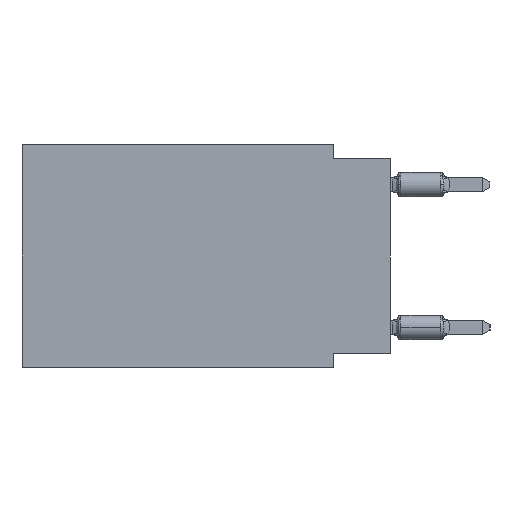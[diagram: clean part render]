
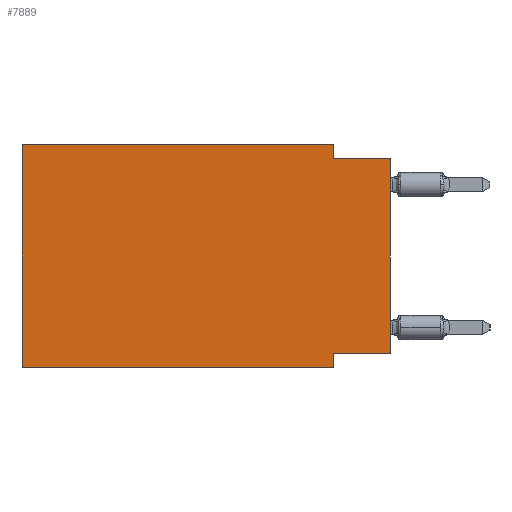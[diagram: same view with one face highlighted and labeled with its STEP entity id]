
A CAD part, left-side view. The second image highlights one B-rep face of the part: STEP entity #7889.
In plain terms, the highlighted planar face has unit normal (-1, 0, 0).
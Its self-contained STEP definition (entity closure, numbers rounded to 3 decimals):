
#257 = LINE ( 'NONE', #14375, #17626 ) ;
#708 = ORIENTED_EDGE ( 'NONE', *, *, #10401, .F. ) ;
#762 = CARTESIAN_POINT ( 'NONE',  ( 0., 16.383, 0. ) ) ;
#1144 = CARTESIAN_POINT ( 'NONE',  ( 0., 0., -9.271 ) ) ;
#1500 = LINE ( 'NONE', #25648, #29223 ) ;
#1559 = DIRECTION ( 'NONE',  ( 0., 0., -1. ) ) ;
#2504 = VERTEX_POINT ( 'NONE', #33860 ) ;
#2645 = VERTEX_POINT ( 'NONE', #31160 ) ;
#3160 = ORIENTED_EDGE ( 'NONE', *, *, #23300, .T. ) ;
#3609 = EDGE_CURVE ( 'NONE', #29315, #2645, #22006, .T. ) ;
#3831 = CARTESIAN_POINT ( 'NONE',  ( 0., 2.54, -9.906 ) ) ;
#3881 = CARTESIAN_POINT ( 'NONE',  ( 0., 16.383, 0. ) ) ;
#4411 = CARTESIAN_POINT ( 'NONE',  ( 0., 0., 0. ) ) ;
#4416 = DIRECTION ( 'NONE',  ( 0., 1., 0. ) ) ;
#4840 = ORIENTED_EDGE ( 'NONE', *, *, #28194, .F. ) ;
#4845 = VERTEX_POINT ( 'NONE', #20992 ) ;
#6410 = LINE ( 'NONE', #20908, #32141 ) ;
#6425 = AXIS2_PLACEMENT_3D ( 'NONE', #18925, #15821, #27598 ) ;
#7889 = ADVANCED_FACE ( 'NONE', ( #9643 ), #15426, .F. ) ;
#7894 = DIRECTION ( 'NONE',  ( 0., 0., 1. ) ) ;
#7958 = EDGE_CURVE ( 'NONE', #2504, #37181, #1500, .T. ) ;
#8965 = ORIENTED_EDGE ( 'NONE', *, *, #26145, .F. ) ;
#9255 = ORIENTED_EDGE ( 'NONE', *, *, #20797, .F. ) ;
#9643 = FACE_OUTER_BOUND ( 'NONE', #13720, .T. ) ;
#10401 = EDGE_CURVE ( 'NONE', #37181, #4845, #36491, .T. ) ;
#10544 = VERTEX_POINT ( 'NONE', #32786 ) ;
#10640 = LINE ( 'NONE', #28403, #34768 ) ;
#10696 = VERTEX_POINT ( 'NONE', #3831 ) ;
#12011 = VECTOR ( 'NONE', #27080, 1000. ) ;
#13720 = EDGE_LOOP ( 'NONE', ( #28308, #9255, #4840, #708, #18012, #3160, #37168, #8965 ) ) ;
#14375 = CARTESIAN_POINT ( 'NONE',  ( 0., 16.383, -9.906 ) ) ;
#15426 = PLANE ( 'NONE',  #6425 ) ;
#15671 = LINE ( 'NONE', #27450, #12011 ) ;
#15821 = DIRECTION ( 'NONE',  ( 1., 0., 0. ) ) ;
#16914 = VERTEX_POINT ( 'NONE', #27980 ) ;
#17626 = VECTOR ( 'NONE', #18049, 1000. ) ;
#18012 = ORIENTED_EDGE ( 'NONE', *, *, #7958, .F. ) ;
#18049 = DIRECTION ( 'NONE',  ( 0., -1., 0. ) ) ;
#18925 = CARTESIAN_POINT ( 'NONE',  ( 0., 16.383, 0. ) ) ;
#20797 = EDGE_CURVE ( 'NONE', #10544, #2645, #15671, .T. ) ;
#20908 = CARTESIAN_POINT ( 'NONE',  ( 0., 2.54, -9.906 ) ) ;
#20992 = CARTESIAN_POINT ( 'NONE',  ( 0., 2.54, 0. ) ) ;
#22006 = LINE ( 'NONE', #4411, #37993 ) ;
#22038 = EDGE_CURVE ( 'NONE', #16914, #10696, #6410, .T. ) ;
#22073 = CARTESIAN_POINT ( 'NONE',  ( 0., 0., -9.271 ) ) ;
#23300 = EDGE_CURVE ( 'NONE', #2504, #10696, #257, .T. ) ;
#25648 = CARTESIAN_POINT ( 'NONE',  ( 0., 16.383, 0. ) ) ;
#26145 = EDGE_CURVE ( 'NONE', #29315, #16914, #30872, .T. ) ;
#26206 = VECTOR ( 'NONE', #27440, 1000. ) ;
#27080 = DIRECTION ( 'NONE',  ( 0., -1., 0. ) ) ;
#27440 = DIRECTION ( 'NONE',  ( 0., -1., 0. ) ) ;
#27450 = CARTESIAN_POINT ( 'NONE',  ( 0., 0., -0.635 ) ) ;
#27598 = DIRECTION ( 'NONE',  ( 0., 0., -1. ) ) ;
#27980 = CARTESIAN_POINT ( 'NONE',  ( 0., 2.54, -9.271 ) ) ;
#28194 = EDGE_CURVE ( 'NONE', #4845, #10544, #10640, .T. ) ;
#28308 = ORIENTED_EDGE ( 'NONE', *, *, #3609, .T. ) ;
#28403 = CARTESIAN_POINT ( 'NONE',  ( 0., 2.54, 0. ) ) ;
#28506 = VECTOR ( 'NONE', #4416, 1000. ) ;
#29223 = VECTOR ( 'NONE', #7894, 1000. ) ;
#29315 = VERTEX_POINT ( 'NONE', #22073 ) ;
#30872 = LINE ( 'NONE', #1144, #28506 ) ;
#31160 = CARTESIAN_POINT ( 'NONE',  ( 0., 0., -0.635 ) ) ;
#32141 = VECTOR ( 'NONE', #32662, 1000. ) ;
#32662 = DIRECTION ( 'NONE',  ( 0., 0., -1. ) ) ;
#32786 = CARTESIAN_POINT ( 'NONE',  ( 0., 2.54, -0.635 ) ) ;
#33764 = DIRECTION ( 'NONE',  ( 0., 0., 1. ) ) ;
#33860 = CARTESIAN_POINT ( 'NONE',  ( 0., 16.383, -9.906 ) ) ;
#34768 = VECTOR ( 'NONE', #1559, 1000. ) ;
#36491 = LINE ( 'NONE', #3881, #26206 ) ;
#37168 = ORIENTED_EDGE ( 'NONE', *, *, #22038, .F. ) ;
#37181 = VERTEX_POINT ( 'NONE', #762 ) ;
#37993 = VECTOR ( 'NONE', #33764, 1000. ) ;
